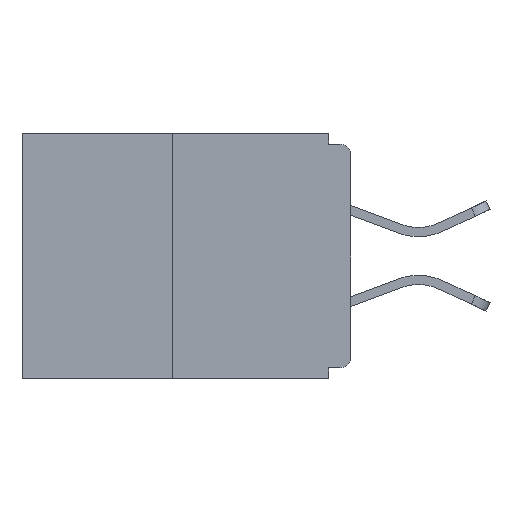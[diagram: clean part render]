
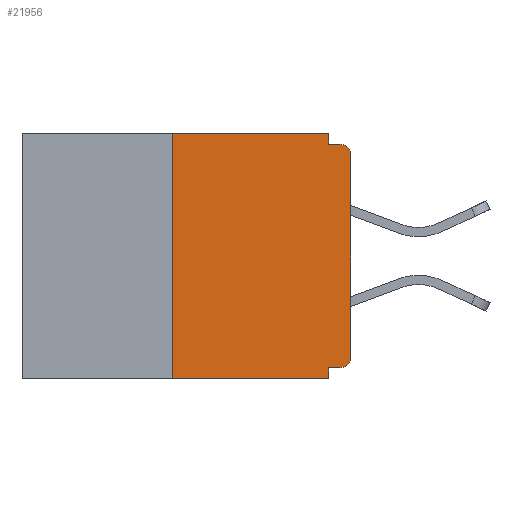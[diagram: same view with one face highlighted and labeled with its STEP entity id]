
A CAD part, left-side view. The second image highlights one B-rep face of the part: STEP entity #21956.
In plain terms, the highlighted planar face has unit normal (-1, 0, 0).
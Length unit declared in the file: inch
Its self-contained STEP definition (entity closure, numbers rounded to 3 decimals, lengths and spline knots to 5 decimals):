
#291 = DIRECTION ( 'NONE',  ( 0., 0., -1. ) ) ;
#984 = ORIENTED_EDGE ( 'NONE', *, *, #3452, .F. ) ;
#1189 = CARTESIAN_POINT ( 'NONE',  ( 0., 0.46, -0.343 ) ) ;
#1667 = DIRECTION ( 'NONE',  ( 0., 0., -1. ) ) ;
#1916 = ORIENTED_EDGE ( 'NONE', *, *, #10808, .T. ) ;
#2186 = CARTESIAN_POINT ( 'NONE',  ( 0., 0.031, -0.328 ) ) ;
#2312 = VERTEX_POINT ( 'NONE', #4024 ) ;
#2498 = EDGE_CURVE ( 'NONE', #18567, #24094, #3450, .T. ) ;
#2935 = LINE ( 'NONE', #18621, #8432 ) ;
#3430 = LINE ( 'NONE', #13051, #9258 ) ;
#3450 = LINE ( 'NONE', #30203, #10409 ) ;
#3452 = EDGE_CURVE ( 'NONE', #25173, #2312, #9601, .T. ) ;
#4024 = CARTESIAN_POINT ( 'NONE',  ( 0., 0.015, -0.015 ) ) ;
#4082 = EDGE_CURVE ( 'NONE', #11020, #21179, #2935, .T. ) ;
#4164 = VECTOR ( 'NONE', #28473, 39.37008 ) ;
#4598 = VERTEX_POINT ( 'NONE', #2186 ) ;
#5091 = CARTESIAN_POINT ( 'NONE',  ( 0., 0., -0.015 ) ) ;
#5216 = VECTOR ( 'NONE', #20132, 39.37008 ) ;
#5295 = CARTESIAN_POINT ( 'NONE',  ( 0., 0.031, -0.015 ) ) ;
#5528 = LINE ( 'NONE', #26857, #21364 ) ;
#5666 = VERTEX_POINT ( 'NONE', #27194 ) ;
#5996 = PLANE ( 'NONE',  #21163 ) ;
#6484 = AXIS2_PLACEMENT_3D ( 'NONE', #11969, #14467, #291 ) ;
#7661 = CARTESIAN_POINT ( 'NONE',  ( 0., 0., -0.313 ) ) ;
#7688 = EDGE_LOOP ( 'NONE', ( #27547, #23093, #1916, #22557, #23472, #19835, #7820, #16256, #984, #23569 ) ) ;
#7820 = ORIENTED_EDGE ( 'NONE', *, *, #4082, .T. ) ;
#7821 = LINE ( 'NONE', #9949, #4164 ) ;
#8432 = VECTOR ( 'NONE', #16930, 39.37008 ) ;
#8591 = VERTEX_POINT ( 'NONE', #17015 ) ;
#9258 = VECTOR ( 'NONE', #1667, 39.37008 ) ;
#9601 = LINE ( 'NONE', #5091, #5216 ) ;
#9949 = CARTESIAN_POINT ( 'NONE',  ( 0., 0.031, 0. ) ) ;
#10234 = CARTESIAN_POINT ( 'NONE',  ( 0., 0., -0.03 ) ) ;
#10409 = VECTOR ( 'NONE', #16040, 39.37008 ) ;
#10701 = DIRECTION ( 'NONE',  ( 0., 0., -1. ) ) ;
#10808 = EDGE_CURVE ( 'NONE', #18567, #28958, #15074, .T. ) ;
#11001 = DIRECTION ( 'NONE',  ( 1., 0., 0. ) ) ;
#11020 = VERTEX_POINT ( 'NONE', #7661 ) ;
#11886 = EDGE_CURVE ( 'NONE', #24094, #8591, #5528, .T. ) ;
#11956 = CARTESIAN_POINT ( 'NONE',  ( 0., 0.25, 0. ) ) ;
#11969 = CARTESIAN_POINT ( 'NONE',  ( 0., 0.015, -0.03 ) ) ;
#12447 = EDGE_CURVE ( 'NONE', #5666, #11020, #26470, .T. ) ;
#12710 = DIRECTION ( 'NONE',  ( 0., -1., 0. ) ) ;
#13051 = CARTESIAN_POINT ( 'NONE',  ( 0., 0.031, -0.343 ) ) ;
#13278 = CIRCLE ( 'NONE', #6484, 0.015 ) ;
#13490 = AXIS2_PLACEMENT_3D ( 'NONE', #24324, #26607, #29116 ) ;
#14467 = DIRECTION ( 'NONE',  ( -1., 0., 0. ) ) ;
#15074 = LINE ( 'NONE', #1189, #26894 ) ;
#15379 = VECTOR ( 'NONE', #20140, 39.37008 ) ;
#16040 = DIRECTION ( 'NONE',  ( 0., 0., 1. ) ) ;
#16256 = ORIENTED_EDGE ( 'NONE', *, *, #18429, .T. ) ;
#16930 = DIRECTION ( 'NONE',  ( 0., 0., 1. ) ) ;
#17015 = CARTESIAN_POINT ( 'NONE',  ( 0., 0.031, 0. ) ) ;
#17668 = CARTESIAN_POINT ( 'NONE',  ( 0., 0., -0.328 ) ) ;
#17880 = CARTESIAN_POINT ( 'NONE',  ( 0., 0.25, -0.343 ) ) ;
#18429 = EDGE_CURVE ( 'NONE', #21179, #2312, #13278, .T. ) ;
#18567 = VERTEX_POINT ( 'NONE', #17880 ) ;
#18621 = CARTESIAN_POINT ( 'NONE',  ( 0., 0., 0. ) ) ;
#19835 = ORIENTED_EDGE ( 'NONE', *, *, #12447, .T. ) ;
#20118 = DIRECTION ( 'NONE',  ( 0., -1., 0. ) ) ;
#20132 = DIRECTION ( 'NONE',  ( 0., -1., 0. ) ) ;
#20136 = FACE_OUTER_BOUND ( 'NONE', #7688, .T. ) ;
#20140 = DIRECTION ( 'NONE',  ( 0., 1., 0. ) ) ;
#21163 = AXIS2_PLACEMENT_3D ( 'NONE', #29626, #11001, #10701 ) ;
#21179 = VERTEX_POINT ( 'NONE', #10234 ) ;
#21364 = VECTOR ( 'NONE', #12710, 39.37008 ) ;
#21956 = ADVANCED_FACE ( 'NONE', ( #20136 ), #5996, .F. ) ;
#22557 = ORIENTED_EDGE ( 'NONE', *, *, #25808, .F. ) ;
#23093 = ORIENTED_EDGE ( 'NONE', *, *, #2498, .F. ) ;
#23472 = ORIENTED_EDGE ( 'NONE', *, *, #29261, .F. ) ;
#23485 = EDGE_CURVE ( 'NONE', #8591, #25173, #7821, .T. ) ;
#23569 = ORIENTED_EDGE ( 'NONE', *, *, #23485, .F. ) ;
#24094 = VERTEX_POINT ( 'NONE', #11956 ) ;
#24324 = CARTESIAN_POINT ( 'NONE',  ( 0., 0.015, -0.313 ) ) ;
#25173 = VERTEX_POINT ( 'NONE', #5295 ) ;
#25808 = EDGE_CURVE ( 'NONE', #4598, #28958, #3430, .T. ) ;
#25916 = CARTESIAN_POINT ( 'NONE',  ( 0., 0.031, -0.343 ) ) ;
#26470 = CIRCLE ( 'NONE', #13490, 0.015 ) ;
#26607 = DIRECTION ( 'NONE',  ( -1., 0., 0. ) ) ;
#26857 = CARTESIAN_POINT ( 'NONE',  ( 0., 0.46, 0. ) ) ;
#26894 = VECTOR ( 'NONE', #20118, 39.37008 ) ;
#27194 = CARTESIAN_POINT ( 'NONE',  ( 0., 0.015, -0.328 ) ) ;
#27547 = ORIENTED_EDGE ( 'NONE', *, *, #11886, .F. ) ;
#28473 = DIRECTION ( 'NONE',  ( 0., 0., -1. ) ) ;
#28958 = VERTEX_POINT ( 'NONE', #25916 ) ;
#29116 = DIRECTION ( 'NONE',  ( 0., 0., -1. ) ) ;
#29261 = EDGE_CURVE ( 'NONE', #5666, #4598, #30537, .T. ) ;
#29626 = CARTESIAN_POINT ( 'NONE',  ( 0., 0.46, 0. ) ) ;
#30203 = CARTESIAN_POINT ( 'NONE',  ( 0., 0.25, 0. ) ) ;
#30537 = LINE ( 'NONE', #17668, #15379 ) ;
